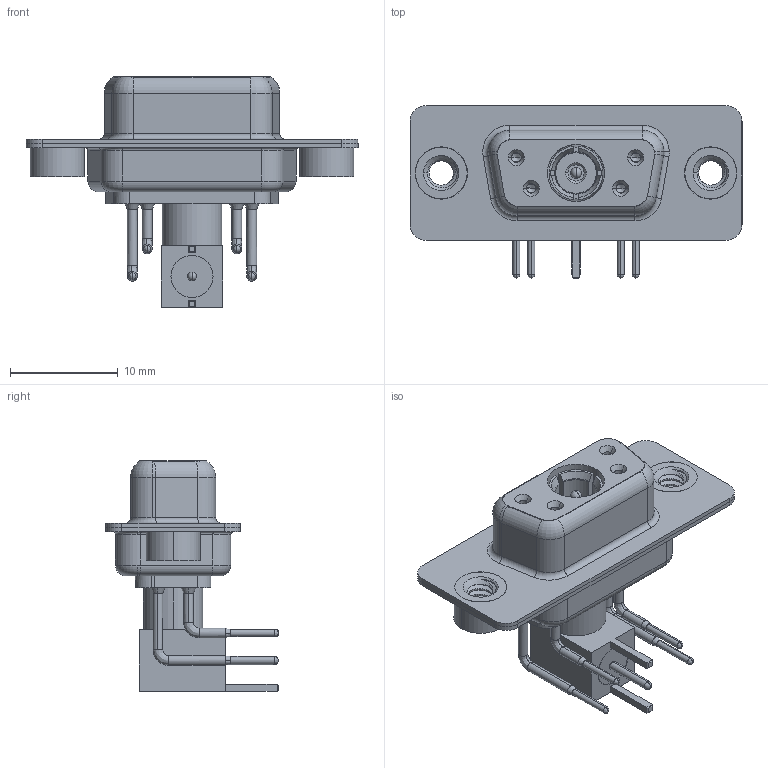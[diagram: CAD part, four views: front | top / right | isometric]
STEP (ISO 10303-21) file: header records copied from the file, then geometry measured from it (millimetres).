
FILE_DESCRIPTION (( 'STEP AP203' ), '1' );
FILE_NAME ('630-5W1-640-5T2.STEP', '2022-05-27T11:49:43', ( '' ), ( '' ), 'SwSTEP 2.0', 'SolidWorks 2020', '' );
FILE_SCHEMA (( 'CONFIG_CONTROL_DESIGN' ));
Length unit declared in the file: millimetre
Products named in the file (14): Pin_RA; Co-Ax Plug_RA PC Tail; 630Combo Contact Row 1; 630Combo Threaded Rivet_2; 630Combo Housing_5W1; 630Combo Contact Row 2; Insulator Pin_Straight PC Tail; Locking Collar; Insulator RA Pin; 630-5W1-640-5T2; 630Combo Shell Front_09 Contacts; Co-Ax Plug Assy_RA; 630Combo Shell Rear_09 Contacts; RA Back Shell
Assembly tree (16 placements, depth 3):
  630-5W1-640-5T2
    630Combo Housing_5W1
    630Combo Shell Front_09 Contacts
    630Combo Shell Rear_09 Contacts
    630Combo Threaded Rivet_2  x2
    Co-Ax Plug Assy_RA
      Co-Ax Plug_RA PC Tail
      Insulator Pin_Straight PC Tail
      Pin_RA
      Locking Collar
      RA Back Shell
      Insulator RA Pin
    630Combo Contact Row 1  x2
    630Combo Contact Row 2  x2
Bounding box: 30.8 x 16 x 21.41 mm (x, y, z)
Volume: 1972.3 mm3; surface area: 5011.9 mm2
Topology: 15 solids, 15 shells, 659 faces, 1626 edges, 1018 vertices
Faces by surface type: cylinder 294, plane 194, cone 81, torus 63, bspline 23, sphere 4
Entity records: 19403 total; most frequent: CARTESIAN_POINT 4775, DIRECTION 2934, ORIENTED_EDGE 2622, EDGE_CURVE 1311, AXIS2_PLACEMENT_3D 1188, VERTEX_POINT 830, CIRCLE 634, EDGE_LOOP 619
